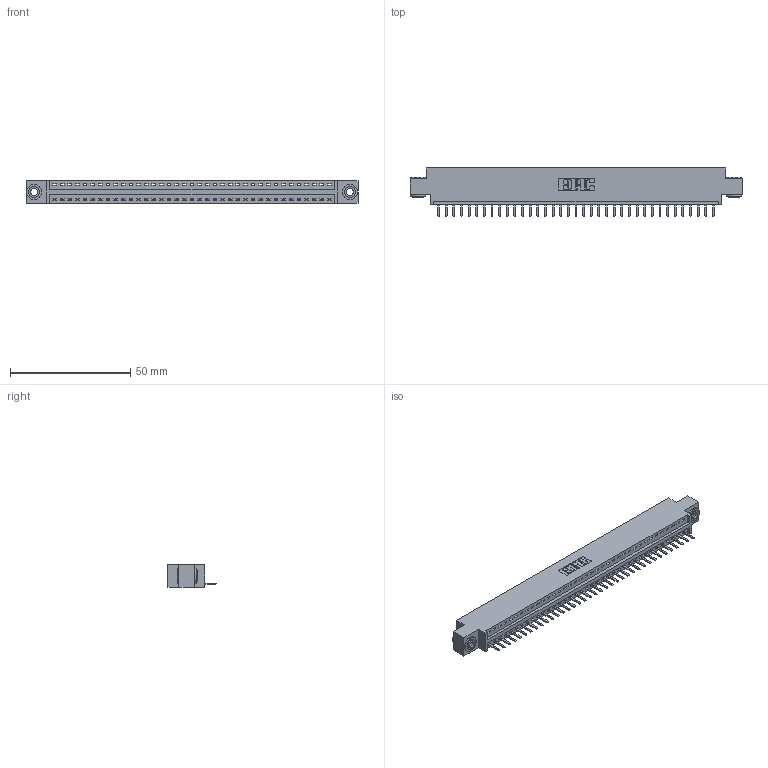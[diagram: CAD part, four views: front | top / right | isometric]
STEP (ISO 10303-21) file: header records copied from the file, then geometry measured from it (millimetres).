
FILE_DESCRIPTION (( 'STEP AP203' ), '1' );
FILE_NAME ('346-037-520-603.STEP', '2022-05-07T02:14:21', ( '' ), ( '' ), 'SwSTEP 2.0', 'SolidWorks 2020', '' );
FILE_SCHEMA (( 'CONFIG_CONTROL_DESIGN' ));
Length unit declared in the file: inch
Products named in the file (4): 345-292-001_345-293-120; 345-250-002_345-250-002-102; 346 Part_0.170 Offset - 0.156 Dia-TH; 346-037-520-603
Assembly tree (40 placements, depth 2):
  346-037-520-603
    346 Part_0.170 Offset - 0.156 Dia-TH
    345-292-001_345-293-120  x37
    345-250-002_345-250-002-102  x2
Bounding box: 138.05 x 20.02 x 9.4 mm (x, y, z)
Volume: 12920.1 mm3; surface area: 16151.1 mm2
Topology: 40 solids, 40 shells, 2472 faces, 7261 edges, 4738 vertices
Faces by surface type: plane 1658, cylinder 806, cone 8
Entity records: 24948 total; most frequent: CARTESIAN_POINT 4272, ORIENTED_EDGE 4222, DIRECTION 3791, EDGE_CURVE 2111, VECTOR 1803, LINE 1803, VERTEX_POINT 1402, AXIS2_PLACEMENT_3D 994
